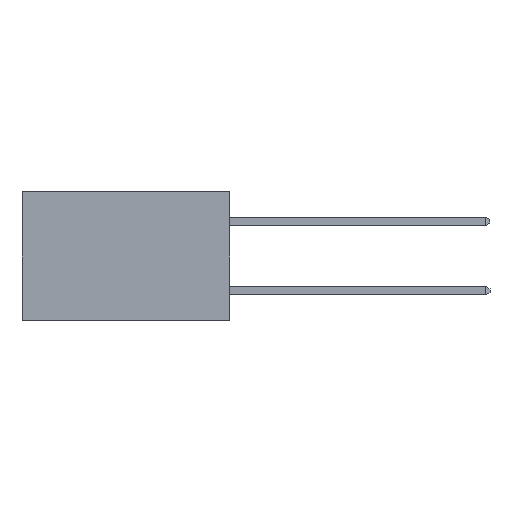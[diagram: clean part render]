
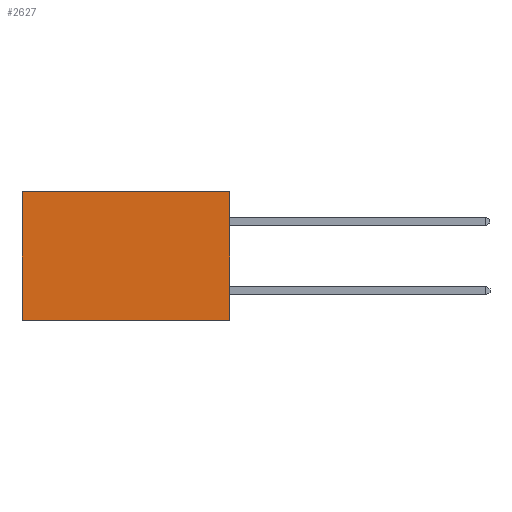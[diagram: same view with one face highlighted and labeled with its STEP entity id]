
A CAD part, left-side view. The second image highlights one B-rep face of the part: STEP entity #2627.
In plain terms, the highlighted planar face has unit normal (-1, 0, 0).
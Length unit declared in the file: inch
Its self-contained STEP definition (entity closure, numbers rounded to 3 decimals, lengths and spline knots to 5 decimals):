
#226 = VERTEX_POINT ( 'NONE', #7740 ) ;
#269 = DIRECTION ( 'NONE',  ( 0., 0., -1. ) ) ;
#322 = DIRECTION ( 'NONE',  ( 1., 0., 0. ) ) ;
#361 = PLANE ( 'NONE',  #7345 ) ;
#370 = VERTEX_POINT ( 'NONE', #2171 ) ;
#502 = CARTESIAN_POINT ( 'NONE',  ( 0.2615, 0., -0.37 ) ) ;
#545 = EDGE_LOOP ( 'NONE', ( #5197, #3727, #5391, #7018 ) ) ;
#750 = LINE ( 'NONE', #4157, #7494 ) ;
#1656 = VERTEX_POINT ( 'NONE', #5980 ) ;
#1797 = DIRECTION ( 'NONE',  ( 0., 0., -1. ) ) ;
#2131 = CARTESIAN_POINT ( 'NONE',  ( 0.2615, 0.6, -0.37 ) ) ;
#2171 = CARTESIAN_POINT ( 'NONE',  ( 0.2615, 0.6, -0.37 ) ) ;
#2627 = ADVANCED_FACE ( 'NONE', ( #5511 ), #361, .F. ) ;
#3181 = EDGE_CURVE ( 'NONE', #226, #370, #750, .T. ) ;
#3295 = VECTOR ( 'NONE', #1797, 39.37008 ) ;
#3648 = DIRECTION ( 'NONE',  ( 0., 1., 0. ) ) ;
#3727 = ORIENTED_EDGE ( 'NONE', *, *, #3181, .F. ) ;
#3780 = LINE ( 'NONE', #5995, #6881 ) ;
#4106 = VECTOR ( 'NONE', #6911, 39.37008 ) ;
#4157 = CARTESIAN_POINT ( 'NONE',  ( 0.2615, 0., -0.37 ) ) ;
#5197 = ORIENTED_EDGE ( 'NONE', *, *, #6685, .T. ) ;
#5391 = ORIENTED_EDGE ( 'NONE', *, *, #7076, .F. ) ;
#5393 = CARTESIAN_POINT ( 'NONE',  ( 0.2615, 0.6, 0. ) ) ;
#5511 = FACE_OUTER_BOUND ( 'NONE', #545, .T. ) ;
#5735 = LINE ( 'NONE', #7028, #4106 ) ;
#5949 = DIRECTION ( 'NONE',  ( 0., 1., 0. ) ) ;
#5980 = CARTESIAN_POINT ( 'NONE',  ( 0.2615, 0., 0. ) ) ;
#5995 = CARTESIAN_POINT ( 'NONE',  ( 0.2615, 0., 0. ) ) ;
#6685 = EDGE_CURVE ( 'NONE', #7239, #370, #8131, .T. ) ;
#6881 = VECTOR ( 'NONE', #5949, 39.37008 ) ;
#6911 = DIRECTION ( 'NONE',  ( 0., 0., -1. ) ) ;
#7018 = ORIENTED_EDGE ( 'NONE', *, *, #7873, .T. ) ;
#7028 = CARTESIAN_POINT ( 'NONE',  ( 0.2615, 0., -0.37 ) ) ;
#7076 = EDGE_CURVE ( 'NONE', #1656, #226, #5735, .T. ) ;
#7239 = VERTEX_POINT ( 'NONE', #5393 ) ;
#7345 = AXIS2_PLACEMENT_3D ( 'NONE', #502, #322, #269 ) ;
#7494 = VECTOR ( 'NONE', #3648, 39.37008 ) ;
#7740 = CARTESIAN_POINT ( 'NONE',  ( 0.2615, 0., -0.37 ) ) ;
#7873 = EDGE_CURVE ( 'NONE', #1656, #7239, #3780, .T. ) ;
#8131 = LINE ( 'NONE', #2131, #3295 ) ;
